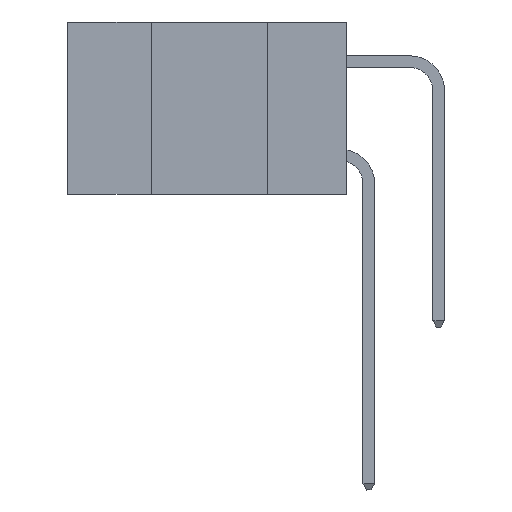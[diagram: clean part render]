
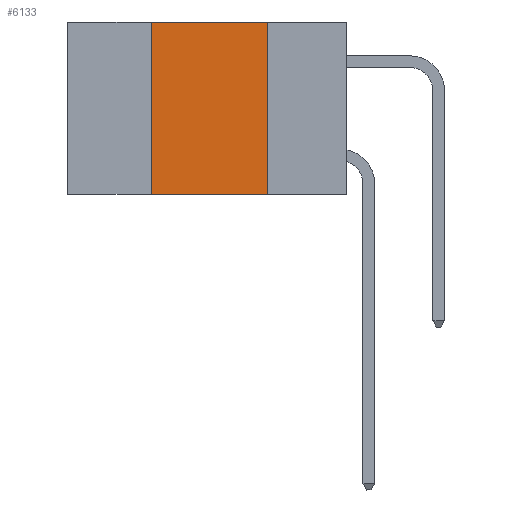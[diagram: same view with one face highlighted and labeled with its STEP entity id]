
A CAD part, left-side view. The second image highlights one B-rep face of the part: STEP entity #6133.
In plain terms, the highlighted planar face has unit normal (-1, 0, 0).
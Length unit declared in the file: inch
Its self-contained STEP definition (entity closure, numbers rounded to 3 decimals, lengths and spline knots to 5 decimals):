
#443 = ORIENTED_EDGE ( 'NONE', *, *, #3267, .F. ) ;
#2015 = ORIENTED_EDGE ( 'NONE', *, *, #4942, .T. ) ;
#2028 = CARTESIAN_POINT ( 'NONE',  ( 0., 0.6, -0.37 ) ) ;
#3201 = VECTOR ( 'NONE', #7023, 39.37008 ) ;
#3267 = EDGE_CURVE ( 'NONE', #11466, #9580, #10334, .T. ) ;
#3630 = PLANE ( 'NONE',  #12751 ) ;
#3807 = CARTESIAN_POINT ( 'NONE',  ( 0., 0.17, 0. ) ) ;
#4374 = VECTOR ( 'NONE', #10623, 39.37008 ) ;
#4649 = CARTESIAN_POINT ( 'NONE',  ( 0., 0.42, 0. ) ) ;
#4942 = EDGE_CURVE ( 'NONE', #11262, #6507, #7719, .T. ) ;
#5029 = DIRECTION ( 'NONE',  ( 0., 0., -1. ) ) ;
#5369 = ORIENTED_EDGE ( 'NONE', *, *, #8055, .F. ) ;
#5808 = CARTESIAN_POINT ( 'NONE',  ( 0., 0.17, 0. ) ) ;
#6082 = DIRECTION ( 'NONE',  ( 1., 0., 0. ) ) ;
#6133 = ADVANCED_FACE ( 'NONE', ( #6818 ), #3630, .F. ) ;
#6507 = VERTEX_POINT ( 'NONE', #7827 ) ;
#6543 = EDGE_LOOP ( 'NONE', ( #5369, #443, #9601, #2015 ) ) ;
#6818 = FACE_OUTER_BOUND ( 'NONE', #6543, .T. ) ;
#7023 = DIRECTION ( 'NONE',  ( 0., 0., 1. ) ) ;
#7719 = LINE ( 'NONE', #2028, #9222 ) ;
#7827 = CARTESIAN_POINT ( 'NONE',  ( 0., 0.17, -0.37 ) ) ;
#8055 = EDGE_CURVE ( 'NONE', #9580, #6507, #12357, .T. ) ;
#8320 = CARTESIAN_POINT ( 'NONE',  ( 0., 0.42, 0. ) ) ;
#9222 = VECTOR ( 'NONE', #12876, 39.37008 ) ;
#9580 = VERTEX_POINT ( 'NONE', #5808 ) ;
#9601 = ORIENTED_EDGE ( 'NONE', *, *, #12618, .F. ) ;
#10334 = LINE ( 'NONE', #11692, #4374 ) ;
#10350 = VECTOR ( 'NONE', #5029, 39.37008 ) ;
#10623 = DIRECTION ( 'NONE',  ( 0., -1., 0. ) ) ;
#11262 = VERTEX_POINT ( 'NONE', #13030 ) ;
#11466 = VERTEX_POINT ( 'NONE', #4649 ) ;
#11543 = DIRECTION ( 'NONE',  ( 0., 0., -1. ) ) ;
#11692 = CARTESIAN_POINT ( 'NONE',  ( 0., 0.6, 0. ) ) ;
#12357 = LINE ( 'NONE', #3807, #10350 ) ;
#12492 = LINE ( 'NONE', #8320, #3201 ) ;
#12618 = EDGE_CURVE ( 'NONE', #11262, #11466, #12492, .T. ) ;
#12751 = AXIS2_PLACEMENT_3D ( 'NONE', #13387, #6082, #11543 ) ;
#12876 = DIRECTION ( 'NONE',  ( 0., -1., 0. ) ) ;
#13030 = CARTESIAN_POINT ( 'NONE',  ( 0., 0.42, -0.37 ) ) ;
#13387 = CARTESIAN_POINT ( 'NONE',  ( 0., 0.6, 0. ) ) ;
